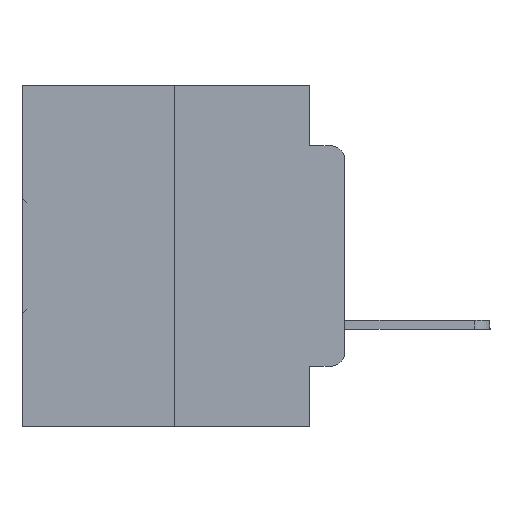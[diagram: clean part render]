
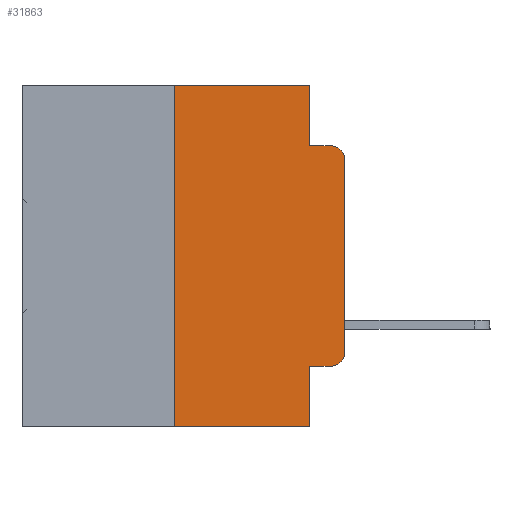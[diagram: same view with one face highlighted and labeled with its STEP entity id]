
A CAD part, left-side view. The second image highlights one B-rep face of the part: STEP entity #31863.
In plain terms, the highlighted planar face has unit normal (-1, 0, 0).
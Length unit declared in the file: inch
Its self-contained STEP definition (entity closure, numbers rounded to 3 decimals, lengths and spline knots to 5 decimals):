
#65 = VECTOR ( 'NONE', #18933, 39.37008 ) ;
#219 = EDGE_CURVE ( 'NONE', #289, #2746, #30911, .T. ) ;
#289 = VERTEX_POINT ( 'NONE', #29557 ) ;
#362 = DIRECTION ( 'NONE',  ( 0., 0., -1. ) ) ;
#876 = CARTESIAN_POINT ( 'NONE',  ( 0., 0.02, -0.1085 ) ) ;
#1488 = LINE ( 'NONE', #24690, #26644 ) ;
#1652 = VECTOR ( 'NONE', #8036, 39.37008 ) ;
#2746 = VERTEX_POINT ( 'NONE', #18285 ) ;
#2900 = DIRECTION ( 'NONE',  ( -1., 0., 0. ) ) ;
#2971 = VERTEX_POINT ( 'NONE', #11973 ) ;
#3232 = FACE_OUTER_BOUND ( 'NONE', #14155, .T. ) ;
#3424 = VERTEX_POINT ( 'NONE', #17178 ) ;
#3696 = CARTESIAN_POINT ( 'NONE',  ( 0., 0.02, -0.4115 ) ) ;
#3746 = DIRECTION ( 'NONE',  ( 1., 0., 0. ) ) ;
#3785 = VERTEX_POINT ( 'NONE', #6809 ) ;
#4641 = AXIS2_PLACEMENT_3D ( 'NONE', #26938, #3746, #13597 ) ;
#4774 = EDGE_CURVE ( 'NONE', #2746, #16026, #8966, .T. ) ;
#5201 = ORIENTED_EDGE ( 'NONE', *, *, #11995, .F. ) ;
#5592 = CARTESIAN_POINT ( 'NONE',  ( 0., 0.02, -0.3915 ) ) ;
#5933 = DIRECTION ( 'NONE',  ( 0., 0., -1. ) ) ;
#6135 = CARTESIAN_POINT ( 'NONE',  ( 0., 0., -0.1085 ) ) ;
#6202 = DIRECTION ( 'NONE',  ( 0., -1., 0. ) ) ;
#6533 = VECTOR ( 'NONE', #19967, 39.37008 ) ;
#6809 = CARTESIAN_POINT ( 'NONE',  ( 0., 0.051, -0.4115 ) ) ;
#7304 = ORIENTED_EDGE ( 'NONE', *, *, #29182, .T. ) ;
#7392 = CARTESIAN_POINT ( 'NONE',  ( 0., 0.051, -0.4115 ) ) ;
#7725 = DIRECTION ( 'NONE',  ( 0., 0., -1. ) ) ;
#8036 = DIRECTION ( 'NONE',  ( 0., -1., 0. ) ) ;
#8183 = AXIS2_PLACEMENT_3D ( 'NONE', #876, #2900, #362 ) ;
#8966 = LINE ( 'NONE', #14067, #24533 ) ;
#9793 = CARTESIAN_POINT ( 'NONE',  ( 0., 0.25, 0. ) ) ;
#10385 = AXIS2_PLACEMENT_3D ( 'NONE', #5592, #31468, #5933 ) ;
#10708 = EDGE_CURVE ( 'NONE', #3785, #29242, #15524, .T. ) ;
#10911 = CIRCLE ( 'NONE', #8183, 0.02 ) ;
#11700 = EDGE_CURVE ( 'NONE', #29242, #27956, #30302, .T. ) ;
#11838 = ORIENTED_EDGE ( 'NONE', *, *, #10708, .T. ) ;
#11973 = CARTESIAN_POINT ( 'NONE',  ( 0., 0.25, 0. ) ) ;
#11995 = EDGE_CURVE ( 'NONE', #15008, #2971, #32982, .T. ) ;
#12028 = DIRECTION ( 'NONE',  ( 0., -1., 0. ) ) ;
#12534 = EDGE_CURVE ( 'NONE', #3785, #3424, #24501, .T. ) ;
#12643 = ORIENTED_EDGE ( 'NONE', *, *, #26073, .T. ) ;
#13597 = DIRECTION ( 'NONE',  ( 0., 0., -1. ) ) ;
#14067 = CARTESIAN_POINT ( 'NONE',  ( 0., 0.051, -0.0885 ) ) ;
#14155 = EDGE_LOOP ( 'NONE', ( #7304, #12643, #19107, #30207, #24189, #5201, #30801, #14724, #11838, #20423 ) ) ;
#14403 = CARTESIAN_POINT ( 'NONE',  ( 0., 0., -0.3915 ) ) ;
#14724 = ORIENTED_EDGE ( 'NONE', *, *, #12534, .F. ) ;
#15008 = VERTEX_POINT ( 'NONE', #29589 ) ;
#15524 = LINE ( 'NONE', #7392, #1652 ) ;
#16026 = VERTEX_POINT ( 'NONE', #17659 ) ;
#16590 = DIRECTION ( 'NONE',  ( 0., 0., 1. ) ) ;
#17178 = CARTESIAN_POINT ( 'NONE',  ( 0., 0.051, -0.5 ) ) ;
#17209 = DIRECTION ( 'NONE',  ( 0., -1., 0. ) ) ;
#17659 = CARTESIAN_POINT ( 'NONE',  ( 0., 0.02, -0.0885 ) ) ;
#18285 = CARTESIAN_POINT ( 'NONE',  ( 0., 0.051, -0.0885 ) ) ;
#18933 = DIRECTION ( 'NONE',  ( 0., 0., -1. ) ) ;
#19107 = ORIENTED_EDGE ( 'NONE', *, *, #4774, .F. ) ;
#19330 = PLANE ( 'NONE',  #4641 ) ;
#19967 = DIRECTION ( 'NONE',  ( 0., 0., 1. ) ) ;
#20199 = VECTOR ( 'NONE', #7725, 39.37008 ) ;
#20423 = ORIENTED_EDGE ( 'NONE', *, *, #11700, .T. ) ;
#24189 = ORIENTED_EDGE ( 'NONE', *, *, #29737, .F. ) ;
#24501 = LINE ( 'NONE', #29086, #65 ) ;
#24533 = VECTOR ( 'NONE', #12028, 39.37008 ) ;
#24690 = CARTESIAN_POINT ( 'NONE',  ( 0., 0., 0. ) ) ;
#24990 = CARTESIAN_POINT ( 'NONE',  ( 0., 0.473, -0.5 ) ) ;
#25090 = VECTOR ( 'NONE', #6202, 39.37008 ) ;
#26073 = EDGE_CURVE ( 'NONE', #32773, #16026, #10911, .T. ) ;
#26644 = VECTOR ( 'NONE', #16590, 39.37008 ) ;
#26845 = CARTESIAN_POINT ( 'NONE',  ( 0., 0.473, 0. ) ) ;
#26938 = CARTESIAN_POINT ( 'NONE',  ( 0., 0.473, 0. ) ) ;
#27293 = VECTOR ( 'NONE', #17209, 39.37008 ) ;
#27511 = LINE ( 'NONE', #24990, #27293 ) ;
#27956 = VERTEX_POINT ( 'NONE', #14403 ) ;
#29061 = LINE ( 'NONE', #26845, #25090 ) ;
#29086 = CARTESIAN_POINT ( 'NONE',  ( 0., 0.051, 0. ) ) ;
#29182 = EDGE_CURVE ( 'NONE', #27956, #32773, #1488, .T. ) ;
#29242 = VERTEX_POINT ( 'NONE', #3696 ) ;
#29557 = CARTESIAN_POINT ( 'NONE',  ( 0., 0.051, 0. ) ) ;
#29589 = CARTESIAN_POINT ( 'NONE',  ( 0., 0.25, -0.5 ) ) ;
#29737 = EDGE_CURVE ( 'NONE', #2971, #289, #29061, .T. ) ;
#30207 = ORIENTED_EDGE ( 'NONE', *, *, #219, .F. ) ;
#30302 = CIRCLE ( 'NONE', #10385, 0.02 ) ;
#30801 = ORIENTED_EDGE ( 'NONE', *, *, #31142, .T. ) ;
#30911 = LINE ( 'NONE', #31245, #20199 ) ;
#31142 = EDGE_CURVE ( 'NONE', #15008, #3424, #27511, .T. ) ;
#31245 = CARTESIAN_POINT ( 'NONE',  ( 0., 0.051, 0. ) ) ;
#31468 = DIRECTION ( 'NONE',  ( -1., 0., 0. ) ) ;
#31863 = ADVANCED_FACE ( 'NONE', ( #3232 ), #19330, .F. ) ;
#32773 = VERTEX_POINT ( 'NONE', #6135 ) ;
#32982 = LINE ( 'NONE', #9793, #6533 ) ;
